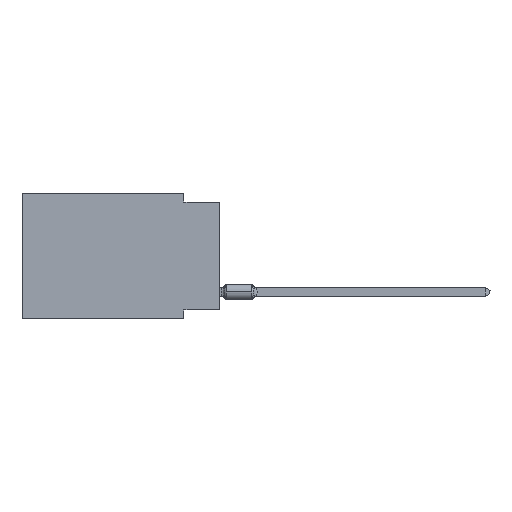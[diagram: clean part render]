
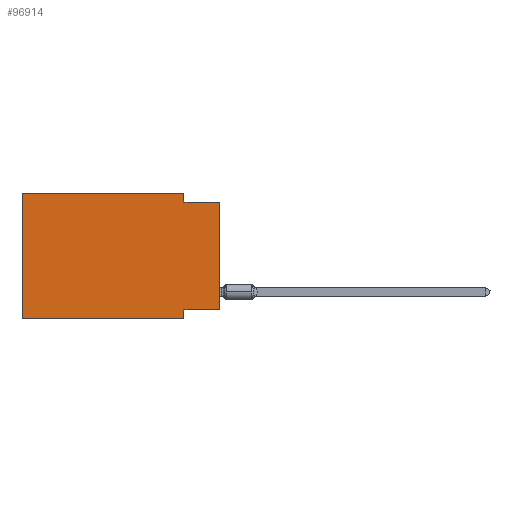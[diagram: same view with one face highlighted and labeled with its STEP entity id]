
A CAD part, left-side view. The second image highlights one B-rep face of the part: STEP entity #96914.
In plain terms, the highlighted planar face has unit normal (-1, 0, 0).
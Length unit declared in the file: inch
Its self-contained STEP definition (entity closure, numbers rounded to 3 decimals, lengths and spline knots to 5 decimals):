
#1287 = CARTESIAN_POINT ( 'NONE',  ( 0., 0.55, 0. ) ) ;
#2153 = DIRECTION ( 'NONE',  ( 0., 0., -1. ) ) ;
#2179 = LINE ( 'NONE', #74300, #89759 ) ;
#4153 = ORIENTED_EDGE ( 'NONE', *, *, #73324, .F. ) ;
#5410 = CARTESIAN_POINT ( 'NONE',  ( 0., 0.55, -0.35 ) ) ;
#6719 = EDGE_CURVE ( 'NONE', #39662, #11951, #41524, .T. ) ;
#11951 = VERTEX_POINT ( 'NONE', #62289 ) ;
#14325 = CARTESIAN_POINT ( 'NONE',  ( 0., 0., -0.325 ) ) ;
#14454 = EDGE_CURVE ( 'NONE', #82461, #11951, #98087, .T. ) ;
#15168 = VECTOR ( 'NONE', #82010, 39.37008 ) ;
#16191 = VERTEX_POINT ( 'NONE', #52012 ) ;
#19229 = DIRECTION ( 'NONE',  ( 0., -1., 0. ) ) ;
#21438 = VERTEX_POINT ( 'NONE', #70211 ) ;
#22688 = VECTOR ( 'NONE', #54746, 39.37008 ) ;
#23072 = CARTESIAN_POINT ( 'NONE',  ( 0., 0.55, 0. ) ) ;
#25021 = VECTOR ( 'NONE', #2153, 39.37008 ) ;
#27564 = AXIS2_PLACEMENT_3D ( 'NONE', #23072, #29301, #44843 ) ;
#28763 = DIRECTION ( 'NONE',  ( 0., -1., 0. ) ) ;
#29301 = DIRECTION ( 'NONE',  ( 1., 0., 0. ) ) ;
#30105 = EDGE_CURVE ( 'NONE', #100870, #21438, #76487, .T. ) ;
#32467 = EDGE_CURVE ( 'NONE', #39662, #53160, #2179, .T. ) ;
#34838 = ORIENTED_EDGE ( 'NONE', *, *, #32467, .F. ) ;
#36296 = CARTESIAN_POINT ( 'NONE',  ( 0., 0.55, 0. ) ) ;
#36543 = LINE ( 'NONE', #68196, #37843 ) ;
#37830 = DIRECTION ( 'NONE',  ( 0., -1., 0. ) ) ;
#37843 = VECTOR ( 'NONE', #52604, 39.37008 ) ;
#39662 = VERTEX_POINT ( 'NONE', #14325 ) ;
#39888 = CARTESIAN_POINT ( 'NONE',  ( 0., 0.55, 0. ) ) ;
#40111 = CARTESIAN_POINT ( 'NONE',  ( 0., 0.1, -0.025 ) ) ;
#41524 = LINE ( 'NONE', #50345, #15168 ) ;
#41599 = DIRECTION ( 'NONE',  ( 0., 1., 0. ) ) ;
#42497 = ORIENTED_EDGE ( 'NONE', *, *, #30105, .T. ) ;
#42692 = EDGE_LOOP ( 'NONE', ( #54696, #97570, #4153, #74667, #46464, #42497, #72861, #34838 ) ) ;
#44843 = DIRECTION ( 'NONE',  ( 0., 0., -1. ) ) ;
#46464 = ORIENTED_EDGE ( 'NONE', *, *, #97463, .F. ) ;
#50345 = CARTESIAN_POINT ( 'NONE',  ( 0., 0., 0. ) ) ;
#52012 = CARTESIAN_POINT ( 'NONE',  ( 0., 0.1, 0. ) ) ;
#52604 = DIRECTION ( 'NONE',  ( 0., 0., -1. ) ) ;
#53160 = VERTEX_POINT ( 'NONE', #53468 ) ;
#53468 = CARTESIAN_POINT ( 'NONE',  ( 0., 0.1, -0.325 ) ) ;
#54696 = ORIENTED_EDGE ( 'NONE', *, *, #6719, .T. ) ;
#54746 = DIRECTION ( 'NONE',  ( 0., 0., 1. ) ) ;
#60144 = LINE ( 'NONE', #36296, #70697 ) ;
#62289 = CARTESIAN_POINT ( 'NONE',  ( 0., 0., -0.025 ) ) ;
#68196 = CARTESIAN_POINT ( 'NONE',  ( 0., 0.1, -0.35 ) ) ;
#70211 = CARTESIAN_POINT ( 'NONE',  ( 0., 0.1, -0.35 ) ) ;
#70697 = VECTOR ( 'NONE', #37830, 39.37008 ) ;
#71360 = LINE ( 'NONE', #1287, #22688 ) ;
#72861 = ORIENTED_EDGE ( 'NONE', *, *, #98924, .F. ) ;
#73324 = EDGE_CURVE ( 'NONE', #16191, #82461, #80514, .T. ) ;
#74300 = CARTESIAN_POINT ( 'NONE',  ( 0., 0., -0.325 ) ) ;
#74667 = ORIENTED_EDGE ( 'NONE', *, *, #83100, .F. ) ;
#75259 = VERTEX_POINT ( 'NONE', #39888 ) ;
#76487 = LINE ( 'NONE', #5410, #84733 ) ;
#80514 = LINE ( 'NONE', #87820, #25021 ) ;
#82010 = DIRECTION ( 'NONE',  ( 0., 0., 1. ) ) ;
#82461 = VERTEX_POINT ( 'NONE', #40111 ) ;
#83100 = EDGE_CURVE ( 'NONE', #75259, #16191, #60144, .T. ) ;
#84013 = VECTOR ( 'NONE', #19229, 39.37008 ) ;
#84733 = VECTOR ( 'NONE', #28763, 39.37008 ) ;
#87820 = CARTESIAN_POINT ( 'NONE',  ( 0., 0.1, 0. ) ) ;
#89759 = VECTOR ( 'NONE', #41599, 39.37008 ) ;
#89792 = CARTESIAN_POINT ( 'NONE',  ( 0., 0., -0.025 ) ) ;
#93652 = PLANE ( 'NONE',  #27564 ) ;
#94156 = FACE_OUTER_BOUND ( 'NONE', #42692, .T. ) ;
#96871 = CARTESIAN_POINT ( 'NONE',  ( 0., 0.55, -0.35 ) ) ;
#96914 = ADVANCED_FACE ( 'NONE', ( #94156 ), #93652, .F. ) ;
#97463 = EDGE_CURVE ( 'NONE', #100870, #75259, #71360, .T. ) ;
#97570 = ORIENTED_EDGE ( 'NONE', *, *, #14454, .F. ) ;
#98087 = LINE ( 'NONE', #89792, #84013 ) ;
#98924 = EDGE_CURVE ( 'NONE', #53160, #21438, #36543, .T. ) ;
#100870 = VERTEX_POINT ( 'NONE', #96871 ) ;
